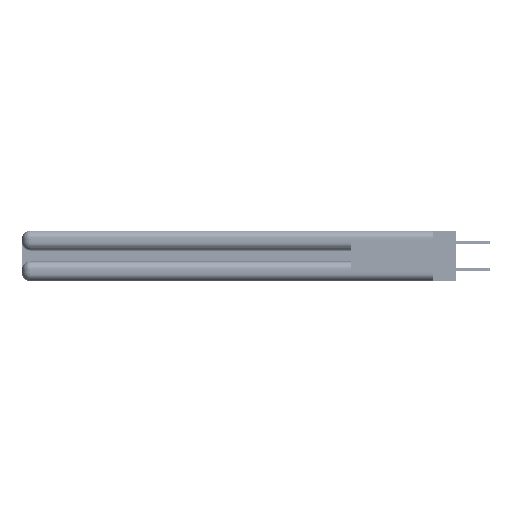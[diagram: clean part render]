
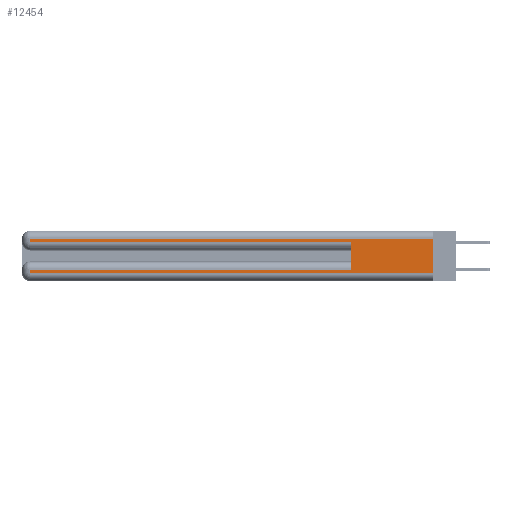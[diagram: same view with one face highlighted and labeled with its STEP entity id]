
A CAD part, left-side view. The second image highlights one B-rep face of the part: STEP entity #12454.
In plain terms, the highlighted planar face has unit normal (-1, 0, 0).
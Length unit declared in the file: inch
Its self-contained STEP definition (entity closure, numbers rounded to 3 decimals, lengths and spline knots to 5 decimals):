
#17 = VECTOR ( 'NONE', #6733, 39.37008 ) ;
#115 = CARTESIAN_POINT ( 'NONE',  ( 0., 0., 0.085 ) ) ;
#960 = VERTEX_POINT ( 'NONE', #16406 ) ;
#2641 = ORIENTED_EDGE ( 'NONE', *, *, #5210, .T. ) ;
#2819 = EDGE_CURVE ( 'NONE', #34713, #36124, #32107, .T. ) ;
#3209 = DIRECTION ( 'NONE',  ( 0., 1., 0. ) ) ;
#5210 = EDGE_CURVE ( 'NONE', #32950, #50002, #13629, .T. ) ;
#6544 = CARTESIAN_POINT ( 'NONE',  ( 0., 2.94, 0.085 ) ) ;
#6733 = DIRECTION ( 'NONE',  ( 0., -1., 0. ) ) ;
#7798 = CARTESIAN_POINT ( 'NONE',  ( 0., 0.6, 0.145 ) ) ;
#8378 = CARTESIAN_POINT ( 'NONE',  ( 0., 2.94, 0.285 ) ) ;
#9176 = VECTOR ( 'NONE', #43915, 39.37008 ) ;
#9578 = DIRECTION ( 'NONE',  ( 1., 0., 0. ) ) ;
#9750 = DIRECTION ( 'NONE',  ( 0., 0., -1. ) ) ;
#10428 = CARTESIAN_POINT ( 'NONE',  ( 0., 0.6, 0.085 ) ) ;
#10992 = VECTOR ( 'NONE', #24500, 39.37008 ) ;
#11865 = CARTESIAN_POINT ( 'NONE',  ( 0., 0., 0.285 ) ) ;
#12454 = ADVANCED_FACE ( 'NONE', ( #22625 ), #39009, .F. ) ;
#13629 = LINE ( 'NONE', #52693, #9176 ) ;
#15639 = VECTOR ( 'NONE', #44797, 39.37008 ) ;
#16257 = EDGE_CURVE ( 'NONE', #27460, #34713, #48238, .T. ) ;
#16406 = CARTESIAN_POINT ( 'NONE',  ( 0., 0., 0.06 ) ) ;
#16977 = CARTESIAN_POINT ( 'NONE',  ( 0., 0., 0.37 ) ) ;
#17255 = CARTESIAN_POINT ( 'NONE',  ( 0., 2.94, 0.37 ) ) ;
#20189 = ORIENTED_EDGE ( 'NONE', *, *, #29154, .F. ) ;
#22029 = EDGE_CURVE ( 'NONE', #39013, #36124, #42683, .T. ) ;
#22625 = FACE_OUTER_BOUND ( 'NONE', #53052, .T. ) ;
#24500 = DIRECTION ( 'NONE',  ( 0., 1., 0. ) ) ;
#24589 = LINE ( 'NONE', #16977, #41950 ) ;
#26716 = EDGE_CURVE ( 'NONE', #39013, #32950, #37979, .T. ) ;
#27047 = CARTESIAN_POINT ( 'NONE',  ( 0., 0.6, 0.285 ) ) ;
#27460 = VERTEX_POINT ( 'NONE', #51283 ) ;
#27586 = EDGE_CURVE ( 'NONE', #50002, #960, #52055, .T. ) ;
#29154 = EDGE_CURVE ( 'NONE', #32974, #960, #24589, .T. ) ;
#29314 = DIRECTION ( 'NONE',  ( 0., 0., -1. ) ) ;
#31110 = ORIENTED_EDGE ( 'NONE', *, *, #27586, .T. ) ;
#32107 = LINE ( 'NONE', #11865, #35294 ) ;
#32124 = VECTOR ( 'NONE', #29314, 39.37008 ) ;
#32950 = VERTEX_POINT ( 'NONE', #6544 ) ;
#32974 = VERTEX_POINT ( 'NONE', #39580 ) ;
#34713 = VERTEX_POINT ( 'NONE', #8378 ) ;
#35080 = ORIENTED_EDGE ( 'NONE', *, *, #22029, .F. ) ;
#35294 = VECTOR ( 'NONE', #50465, 39.37008 ) ;
#35774 = ORIENTED_EDGE ( 'NONE', *, *, #45935, .T. ) ;
#36124 = VERTEX_POINT ( 'NONE', #27047 ) ;
#36903 = AXIS2_PLACEMENT_3D ( 'NONE', #50702, #9578, #9750 ) ;
#37476 = DIRECTION ( 'NONE',  ( 0., 0., -1. ) ) ;
#37979 = LINE ( 'NONE', #115, #10992 ) ;
#38607 = CARTESIAN_POINT ( 'NONE',  ( 0., 2.94, 0.06 ) ) ;
#39009 = PLANE ( 'NONE',  #36903 ) ;
#39013 = VERTEX_POINT ( 'NONE', #10428 ) ;
#39580 = CARTESIAN_POINT ( 'NONE',  ( 0., 0., 0.31 ) ) ;
#39945 = CARTESIAN_POINT ( 'NONE',  ( 0., 0., 0.06 ) ) ;
#40183 = CARTESIAN_POINT ( 'NONE',  ( 0., 0., 0.31 ) ) ;
#41950 = VECTOR ( 'NONE', #37476, 39.37008 ) ;
#42683 = LINE ( 'NONE', #7798, #15639 ) ;
#43915 = DIRECTION ( 'NONE',  ( 0., 0., -1. ) ) ;
#44352 = ORIENTED_EDGE ( 'NONE', *, *, #2819, .T. ) ;
#44797 = DIRECTION ( 'NONE',  ( 0., 0., 1. ) ) ;
#45935 = EDGE_CURVE ( 'NONE', #32974, #27460, #46448, .T. ) ;
#46448 = LINE ( 'NONE', #40183, #49644 ) ;
#48238 = LINE ( 'NONE', #17255, #32124 ) ;
#48368 = ORIENTED_EDGE ( 'NONE', *, *, #26716, .T. ) ;
#49644 = VECTOR ( 'NONE', #3209, 39.37008 ) ;
#50002 = VERTEX_POINT ( 'NONE', #38607 ) ;
#50465 = DIRECTION ( 'NONE',  ( 0., -1., 0. ) ) ;
#50702 = CARTESIAN_POINT ( 'NONE',  ( 0., 0., 0.37 ) ) ;
#51283 = CARTESIAN_POINT ( 'NONE',  ( 0., 2.94, 0.31 ) ) ;
#52055 = LINE ( 'NONE', #39945, #17 ) ;
#52154 = ORIENTED_EDGE ( 'NONE', *, *, #16257, .T. ) ;
#52693 = CARTESIAN_POINT ( 'NONE',  ( 0., 2.94, 0.37 ) ) ;
#53052 = EDGE_LOOP ( 'NONE', ( #20189, #35774, #52154, #44352, #35080, #48368, #2641, #31110 ) ) ;
